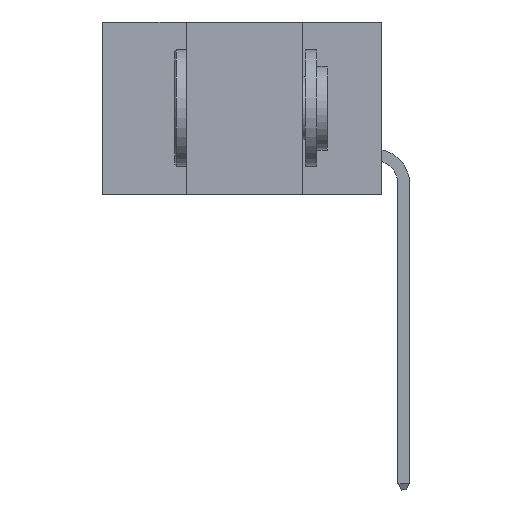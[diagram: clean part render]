
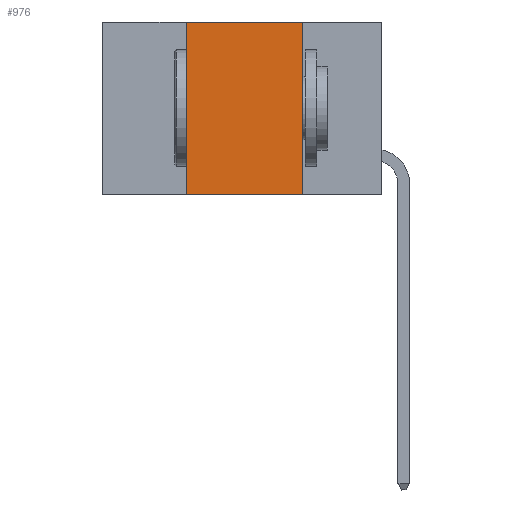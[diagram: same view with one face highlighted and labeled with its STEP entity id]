
A CAD part, left-side view. The second image highlights one B-rep face of the part: STEP entity #976.
In plain terms, the highlighted planar face has unit normal (-1, 0, 0).
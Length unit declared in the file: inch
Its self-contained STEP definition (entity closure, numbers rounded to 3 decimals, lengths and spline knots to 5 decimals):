
#976 = ADVANCED_FACE ( 'NONE', ( #28526 ), #1990, .F. ) ;
#1618 = EDGE_CURVE ( 'NONE', #45576, #35274, #11191, .T. ) ;
#1990 = PLANE ( 'NONE',  #28960 ) ;
#2488 = ORIENTED_EDGE ( 'NONE', *, *, #35995, .F. ) ;
#4795 = DIRECTION ( 'NONE',  ( 0., -1., 0. ) ) ;
#8084 = VECTOR ( 'NONE', #12172, 39.37008 ) ;
#8350 = VECTOR ( 'NONE', #4795, 39.37008 ) ;
#9195 = VERTEX_POINT ( 'NONE', #15410 ) ;
#11169 = ORIENTED_EDGE ( 'NONE', *, *, #1618, .F. ) ;
#11191 = LINE ( 'NONE', #12218, #17321 ) ;
#12172 = DIRECTION ( 'NONE',  ( 0., 0., -1. ) ) ;
#12218 = CARTESIAN_POINT ( 'NONE',  ( 0., 0.42, 0. ) ) ;
#15410 = CARTESIAN_POINT ( 'NONE',  ( 0., 0.17, -0.37 ) ) ;
#15483 = ORIENTED_EDGE ( 'NONE', *, *, #30373, .T. ) ;
#16307 = DIRECTION ( 'NONE',  ( 1., 0., 0. ) ) ;
#17321 = VECTOR ( 'NONE', #34402, 39.37008 ) ;
#22578 = LINE ( 'NONE', #36901, #8084 ) ;
#28526 = FACE_OUTER_BOUND ( 'NONE', #38447, .T. ) ;
#28893 = CARTESIAN_POINT ( 'NONE',  ( 0., 0.17, 0. ) ) ;
#28960 = AXIS2_PLACEMENT_3D ( 'NONE', #34463, #16307, #45349 ) ;
#30373 = EDGE_CURVE ( 'NONE', #45576, #9195, #44787, .T. ) ;
#30610 = LINE ( 'NONE', #42443, #8350 ) ;
#33109 = CARTESIAN_POINT ( 'NONE',  ( 0., 0.42, -0.37 ) ) ;
#33756 = CARTESIAN_POINT ( 'NONE',  ( 0., 0.6, -0.37 ) ) ;
#34402 = DIRECTION ( 'NONE',  ( 0., 0., 1. ) ) ;
#34463 = CARTESIAN_POINT ( 'NONE',  ( 0., 0.6, 0. ) ) ;
#35274 = VERTEX_POINT ( 'NONE', #45910 ) ;
#35995 = EDGE_CURVE ( 'NONE', #35274, #38935, #30610, .T. ) ;
#36901 = CARTESIAN_POINT ( 'NONE',  ( 0., 0.17, 0. ) ) ;
#38447 = EDGE_LOOP ( 'NONE', ( #40186, #2488, #11169, #15483 ) ) ;
#38935 = VERTEX_POINT ( 'NONE', #28893 ) ;
#40186 = ORIENTED_EDGE ( 'NONE', *, *, #42960, .F. ) ;
#40631 = DIRECTION ( 'NONE',  ( 0., -1., 0. ) ) ;
#42443 = CARTESIAN_POINT ( 'NONE',  ( 0., 0.6, 0. ) ) ;
#42573 = VECTOR ( 'NONE', #40631, 39.37008 ) ;
#42960 = EDGE_CURVE ( 'NONE', #38935, #9195, #22578, .T. ) ;
#44787 = LINE ( 'NONE', #33756, #42573 ) ;
#45349 = DIRECTION ( 'NONE',  ( 0., 0., -1. ) ) ;
#45576 = VERTEX_POINT ( 'NONE', #33109 ) ;
#45910 = CARTESIAN_POINT ( 'NONE',  ( 0., 0.42, 0. ) ) ;
